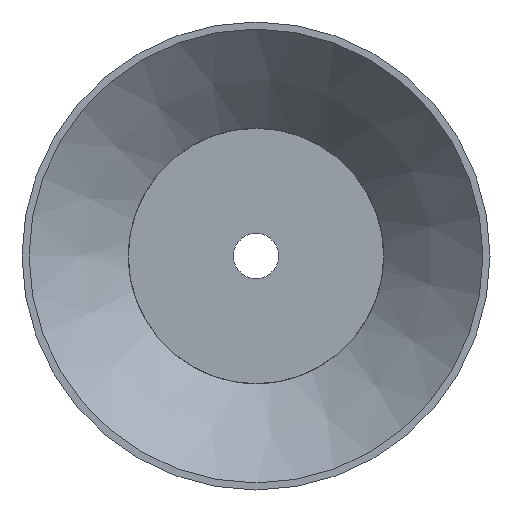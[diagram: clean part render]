
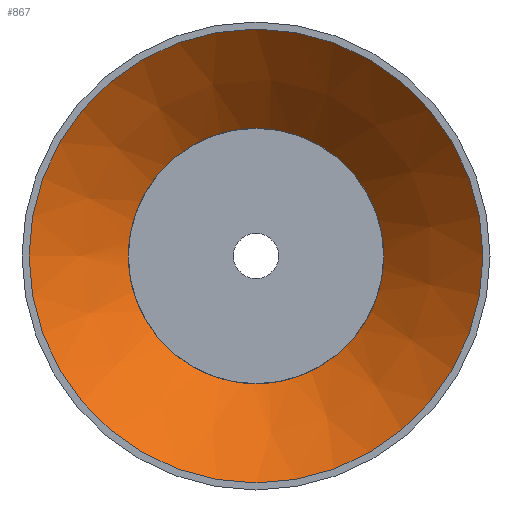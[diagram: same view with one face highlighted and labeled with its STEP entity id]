
A CAD part, front view. The second image highlights one B-rep face of the part: STEP entity #867.
In plain terms, the highlighted conical face has half-angle 45.227 degrees and reference radius 31.679 mm.
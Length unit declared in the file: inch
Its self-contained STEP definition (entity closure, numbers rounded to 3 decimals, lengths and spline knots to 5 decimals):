
#100=(
BOUNDED_CURVE()
B_SPLINE_CURVE(2,(#1198,#1199,#1200),.UNSPECIFIED.,.F.,.F.)
B_SPLINE_CURVE_WITH_KNOTS((3,3),(0.,0.0225),.UNSPECIFIED.)
CURVE()
GEOMETRIC_REPRESENTATION_ITEM()
RATIONAL_B_SPLINE_CURVE((1.,1.,1.))
REPRESENTATION_ITEM('')
);
#101=(
BOUNDED_CURVE()
B_SPLINE_CURVE(2,(#1202,#1203,#1204),.UNSPECIFIED.,.F.,.F.)
B_SPLINE_CURVE_WITH_KNOTS((3,3),(0.84945,0.87196),
 .UNSPECIFIED.)
CURVE()
GEOMETRIC_REPRESENTATION_ITEM()
RATIONAL_B_SPLINE_CURVE((1.,1.,1.))
REPRESENTATION_ITEM('')
);
#102=(
BOUNDED_CURVE()
B_SPLINE_CURVE(2,(#1207,#1208,#1209),.UNSPECIFIED.,.F.,.F.)
B_SPLINE_CURVE_WITH_KNOTS((3,3),(0.,0.0225),.UNSPECIFIED.)
CURVE()
GEOMETRIC_REPRESENTATION_ITEM()
RATIONAL_B_SPLINE_CURVE((1.,1.,1.))
REPRESENTATION_ITEM('')
);
#103=(
BOUNDED_CURVE()
B_SPLINE_CURVE(2,(#1211,#1212,#1213),.UNSPECIFIED.,.F.,.F.)
B_SPLINE_CURVE_WITH_KNOTS((3,3),(0.84929,0.87179),
 .UNSPECIFIED.)
CURVE()
GEOMETRIC_REPRESENTATION_ITEM()
RATIONAL_B_SPLINE_CURVE((1.,1.,1.))
REPRESENTATION_ITEM('')
);
#104=(
BOUNDED_CURVE()
B_SPLINE_CURVE(2,(#1216,#1217,#1218),.UNSPECIFIED.,.F.,.F.)
B_SPLINE_CURVE_WITH_KNOTS((3,3),(0.,0.0225),.UNSPECIFIED.)
CURVE()
GEOMETRIC_REPRESENTATION_ITEM()
RATIONAL_B_SPLINE_CURVE((1.,1.,1.))
REPRESENTATION_ITEM('')
);
#105=(
BOUNDED_CURVE()
B_SPLINE_CURVE(2,(#1220,#1221,#1222),.UNSPECIFIED.,.F.,.F.)
B_SPLINE_CURVE_WITH_KNOTS((3,3),(0.84951,0.87201),
 .UNSPECIFIED.)
CURVE()
GEOMETRIC_REPRESENTATION_ITEM()
RATIONAL_B_SPLINE_CURVE((1.,1.,1.))
REPRESENTATION_ITEM('')
);
#106=(
BOUNDED_CURVE()
B_SPLINE_CURVE(2,(#1225,#1226,#1227),.UNSPECIFIED.,.F.,.F.)
B_SPLINE_CURVE_WITH_KNOTS((3,3),(0.,0.0225),.UNSPECIFIED.)
CURVE()
GEOMETRIC_REPRESENTATION_ITEM()
RATIONAL_B_SPLINE_CURVE((1.,1.,1.))
REPRESENTATION_ITEM('')
);
#107=(
BOUNDED_CURVE()
B_SPLINE_CURVE(2,(#1229,#1230,#1231),.UNSPECIFIED.,.F.,.F.)
B_SPLINE_CURVE_WITH_KNOTS((3,3),(0.8493,0.8718),
 .UNSPECIFIED.)
CURVE()
GEOMETRIC_REPRESENTATION_ITEM()
RATIONAL_B_SPLINE_CURVE((1.,1.,1.))
REPRESENTATION_ITEM('')
);
#130=CONICAL_SURFACE('',#935,1.24721,0.789);
#137=FACE_OUTER_BOUND('',#179,.T.);
#179=EDGE_LOOP('',(#586,#587,#588,#589,#590,#591,#592,#593,#594,#595,#596,
#597,#598,#599,#600,#601,#602,#603,#604,#605,#606));
#218=CIRCLE('',#918,0.89443);
#219=CIRCLE('',#920,0.89443);
#221=CIRCLE('',#923,0.89443);
#224=CIRCLE('',#927,0.89443);
#228=CIRCLE('',#933,1.6);
#229=CIRCLE('',#934,1.6);
#230=CIRCLE('',#936,0.9);
#231=CIRCLE('',#937,0.9);
#232=CIRCLE('',#938,0.9);
#233=CIRCLE('',#939,0.9);
#234=CIRCLE('',#940,0.9);
#263=LINE('',#1195,#293);
#293=VECTOR('',#1032,1.24721);
#315=VERTEX_POINT('',#1146);
#317=VERTEX_POINT('',#1150);
#318=VERTEX_POINT('',#1154);
#320=VERTEX_POINT('',#1157);
#322=VERTEX_POINT('',#1163);
#324=VERTEX_POINT('',#1166);
#327=VERTEX_POINT('',#1173);
#329=VERTEX_POINT('',#1177);
#333=VERTEX_POINT('',#1189);
#334=VERTEX_POINT('',#1190);
#335=VERTEX_POINT('',#1194);
#336=VERTEX_POINT('',#1196);
#337=VERTEX_POINT('',#1201);
#338=VERTEX_POINT('',#1205);
#339=VERTEX_POINT('',#1210);
#340=VERTEX_POINT('',#1214);
#341=VERTEX_POINT('',#1219);
#342=VERTEX_POINT('',#1223);
#343=VERTEX_POINT('',#1228);
#418=EDGE_CURVE('',#317,#315,#218,.T.);
#420=EDGE_CURVE('',#318,#320,#219,.T.);
#424=EDGE_CURVE('',#322,#324,#221,.T.);
#430=EDGE_CURVE('',#329,#327,#224,.T.);
#435=EDGE_CURVE('',#333,#334,#228,.T.);
#436=EDGE_CURVE('',#334,#333,#229,.T.);
#437=EDGE_CURVE('',#334,#335,#263,.T.);
#438=EDGE_CURVE('',#336,#335,#230,.T.);
#439=EDGE_CURVE('',#327,#336,#100,.T.);
#440=EDGE_CURVE('',#337,#329,#101,.T.);
#441=EDGE_CURVE('',#338,#337,#231,.T.);
#442=EDGE_CURVE('',#315,#338,#102,.T.);
#443=EDGE_CURVE('',#339,#317,#103,.T.);
#444=EDGE_CURVE('',#340,#339,#232,.T.);
#445=EDGE_CURVE('',#320,#340,#104,.T.);
#446=EDGE_CURVE('',#341,#318,#105,.T.);
#447=EDGE_CURVE('',#342,#341,#233,.T.);
#448=EDGE_CURVE('',#324,#342,#106,.T.);
#449=EDGE_CURVE('',#343,#322,#107,.T.);
#450=EDGE_CURVE('',#335,#343,#234,.T.);
#586=ORIENTED_EDGE('',*,*,#435,.T.);
#587=ORIENTED_EDGE('',*,*,#437,.T.);
#588=ORIENTED_EDGE('',*,*,#438,.F.);
#589=ORIENTED_EDGE('',*,*,#439,.F.);
#590=ORIENTED_EDGE('',*,*,#430,.F.);
#591=ORIENTED_EDGE('',*,*,#440,.F.);
#592=ORIENTED_EDGE('',*,*,#441,.F.);
#593=ORIENTED_EDGE('',*,*,#442,.F.);
#594=ORIENTED_EDGE('',*,*,#418,.F.);
#595=ORIENTED_EDGE('',*,*,#443,.F.);
#596=ORIENTED_EDGE('',*,*,#444,.F.);
#597=ORIENTED_EDGE('',*,*,#445,.F.);
#598=ORIENTED_EDGE('',*,*,#420,.F.);
#599=ORIENTED_EDGE('',*,*,#446,.F.);
#600=ORIENTED_EDGE('',*,*,#447,.F.);
#601=ORIENTED_EDGE('',*,*,#448,.F.);
#602=ORIENTED_EDGE('',*,*,#424,.F.);
#603=ORIENTED_EDGE('',*,*,#449,.F.);
#604=ORIENTED_EDGE('',*,*,#450,.F.);
#605=ORIENTED_EDGE('',*,*,#437,.F.);
#606=ORIENTED_EDGE('',*,*,#436,.T.);
#867=ADVANCED_FACE('',(#137),#130,.F.);
#918=AXIS2_PLACEMENT_3D('',#1152,#989,#990);
#920=AXIS2_PLACEMENT_3D('',#1158,#994,#995);
#923=AXIS2_PLACEMENT_3D('',#1167,#1002,#1003);
#927=AXIS2_PLACEMENT_3D('',#1179,#1013,#1014);
#933=AXIS2_PLACEMENT_3D('',#1191,#1026,#1027);
#934=AXIS2_PLACEMENT_3D('',#1192,#1028,#1029);
#935=AXIS2_PLACEMENT_3D('',#1193,#1030,#1031);
#936=AXIS2_PLACEMENT_3D('',#1197,#1033,#1034);
#937=AXIS2_PLACEMENT_3D('',#1206,#1035,#1036);
#938=AXIS2_PLACEMENT_3D('',#1215,#1037,#1038);
#939=AXIS2_PLACEMENT_3D('',#1224,#1039,#1040);
#940=AXIS2_PLACEMENT_3D('',#1232,#1041,#1042);
#989=DIRECTION('center_axis',(0.,-1.,0.));
#990=DIRECTION('ref_axis',(1.,0.,0.));
#994=DIRECTION('center_axis',(0.,-1.,0.));
#995=DIRECTION('ref_axis',(1.,0.,0.));
#1002=DIRECTION('center_axis',(0.,-1.,0.));
#1003=DIRECTION('ref_axis',(1.,0.,0.));
#1013=DIRECTION('center_axis',(0.,-1.,0.));
#1014=DIRECTION('ref_axis',(1.,0.,0.));
#1026=DIRECTION('center_axis',(0.,-1.,0.));
#1027=DIRECTION('ref_axis',(1.,0.,0.));
#1028=DIRECTION('center_axis',(0.,-1.,0.));
#1029=DIRECTION('ref_axis',(1.,0.,0.));
#1030=DIRECTION('center_axis',(0.,-1.,0.));
#1031=DIRECTION('ref_axis',(1.,0.,0.));
#1032=DIRECTION('',(0.71,0.704,0.));
#1033=DIRECTION('center_axis',(0.,-1.,0.));
#1034=DIRECTION('ref_axis',(1.,0.,0.));
#1035=DIRECTION('center_axis',(0.,-1.,0.));
#1036=DIRECTION('ref_axis',(1.,0.,0.));
#1037=DIRECTION('center_axis',(0.,-1.,0.));
#1038=DIRECTION('ref_axis',(1.,0.,0.));
#1039=DIRECTION('center_axis',(0.,-1.,0.));
#1040=DIRECTION('ref_axis',(1.,0.,0.));
#1041=DIRECTION('center_axis',(0.,-1.,0.));
#1042=DIRECTION('ref_axis',(1.,0.,0.));
#1146=CARTESIAN_POINT('',(0.09993,0.7,0.88883));
#1150=CARTESIAN_POINT('',(0.88882,0.7,0.1));
#1152=CARTESIAN_POINT('Origin',(0.,0.7,0.));
#1154=CARTESIAN_POINT('',(0.09981,0.7,-0.88884));
#1157=CARTESIAN_POINT('',(0.88882,0.7,-0.1));
#1158=CARTESIAN_POINT('Origin',(0.,0.7,0.));
#1163=CARTESIAN_POINT('',(-0.88882,0.7,-0.09999));
#1166=CARTESIAN_POINT('',(-0.1001,0.7,-0.88881));
#1167=CARTESIAN_POINT('Origin',(0.,0.7,0.));
#1173=CARTESIAN_POINT('',(-0.88882,0.7,0.09999));
#1177=CARTESIAN_POINT('',(-0.09986,0.7,0.88884));
#1179=CARTESIAN_POINT('Origin',(0.,0.7,0.));
#1189=CARTESIAN_POINT('',(1.6,0.,0.));
#1190=CARTESIAN_POINT('',(-1.6,0.,0.));
#1191=CARTESIAN_POINT('Origin',(0.,0.,0.));
#1192=CARTESIAN_POINT('Origin',(0.,0.,0.));
#1193=CARTESIAN_POINT('Origin',(0.,0.35,0.));
#1194=CARTESIAN_POINT('',(-0.9,0.69447,0.));
#1195=CARTESIAN_POINT('',(-1.24721,0.35,0.));
#1196=CARTESIAN_POINT('',(-0.89443,0.69447,0.09999));
#1197=CARTESIAN_POINT('Origin',(0.,0.69447,0.));
#1198=CARTESIAN_POINT('Ctrl Pts',(-0.88882,0.7,
0.09999));
#1199=CARTESIAN_POINT('Ctrl Pts',(-0.89162,0.69724,
0.09999));
#1200=CARTESIAN_POINT('Ctrl Pts',(-0.89443,0.69447,
0.09999));
#1201=CARTESIAN_POINT('',(-0.09986,0.69447,0.89444));
#1202=CARTESIAN_POINT('Ctrl Pts',(-0.09986,0.69447,
0.89444));
#1203=CARTESIAN_POINT('Ctrl Pts',(-0.09986,0.69724,
0.89163));
#1204=CARTESIAN_POINT('Ctrl Pts',(-0.09986,0.7,
0.88884));
#1205=CARTESIAN_POINT('',(0.09992,0.69447,0.89444));
#1206=CARTESIAN_POINT('Origin',(0.,0.69447,0.));
#1207=CARTESIAN_POINT('Ctrl Pts',(0.09993,0.7,
0.88883));
#1208=CARTESIAN_POINT('Ctrl Pts',(0.09992,0.69724,0.89162));
#1209=CARTESIAN_POINT('Ctrl Pts',(0.09992,0.69447,
0.89444));
#1210=CARTESIAN_POINT('',(0.89443,0.69447,0.1));
#1211=CARTESIAN_POINT('Ctrl Pts',(0.89443,0.69447,0.1));
#1212=CARTESIAN_POINT('Ctrl Pts',(0.89161,0.69724,0.1));
#1213=CARTESIAN_POINT('Ctrl Pts',(0.88882,0.7,0.1));
#1214=CARTESIAN_POINT('',(0.89443,0.69447,-0.1));
#1215=CARTESIAN_POINT('Origin',(0.,0.69447,0.));
#1216=CARTESIAN_POINT('Ctrl Pts',(0.88882,0.7,-0.1));
#1217=CARTESIAN_POINT('Ctrl Pts',(0.89161,0.69724,-0.1));
#1218=CARTESIAN_POINT('Ctrl Pts',(0.89443,0.69447,-0.1));
#1219=CARTESIAN_POINT('',(0.09981,0.69447,-0.89445));
#1220=CARTESIAN_POINT('Ctrl Pts',(0.09981,0.69447,
-0.89445));
#1221=CARTESIAN_POINT('Ctrl Pts',(0.09981,0.69724,
-0.89164));
#1222=CARTESIAN_POINT('Ctrl Pts',(0.09981,0.7,
-0.88884));
#1223=CARTESIAN_POINT('',(-0.1001,0.69447,-0.89442));
#1224=CARTESIAN_POINT('Origin',(0.,0.69447,0.));
#1225=CARTESIAN_POINT('Ctrl Pts',(-0.1001,0.7,
-0.88881));
#1226=CARTESIAN_POINT('Ctrl Pts',(-0.1001,0.69724,
-0.8916));
#1227=CARTESIAN_POINT('Ctrl Pts',(-0.1001,0.69447,-0.89442));
#1228=CARTESIAN_POINT('',(-0.89443,0.69447,-0.09999));
#1229=CARTESIAN_POINT('Ctrl Pts',(-0.89443,0.69447,
-0.09999));
#1230=CARTESIAN_POINT('Ctrl Pts',(-0.89162,0.69724,
-0.09999));
#1231=CARTESIAN_POINT('Ctrl Pts',(-0.88882,0.7,-0.09999));
#1232=CARTESIAN_POINT('Origin',(0.,0.69447,0.));
